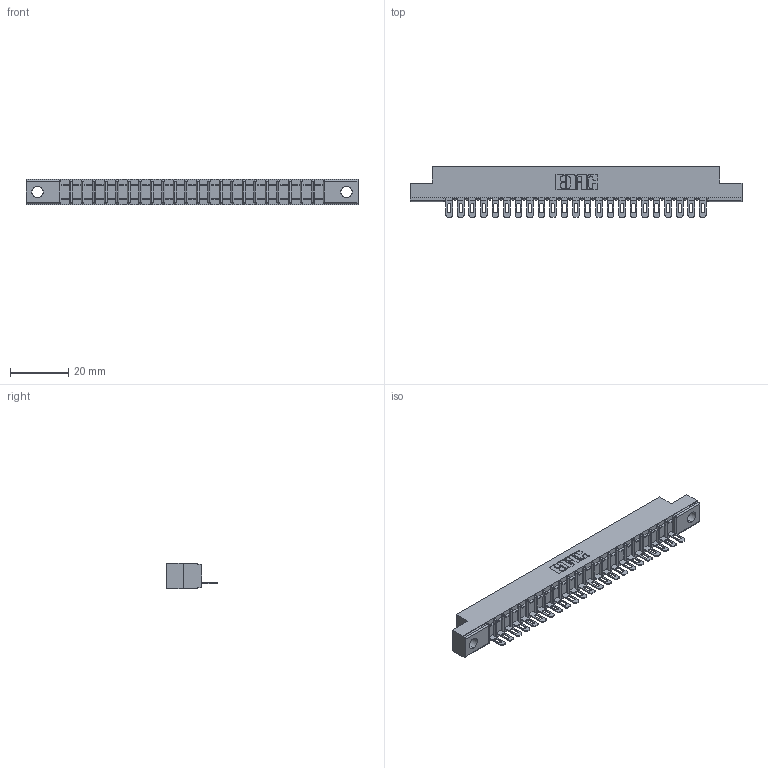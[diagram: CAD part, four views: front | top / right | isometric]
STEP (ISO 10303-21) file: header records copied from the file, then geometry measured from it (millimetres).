
FILE_DESCRIPTION (( 'STEP AP203' ), '1' );
FILE_NAME ('357-023-401-104.STEP', '2020-10-01T10:57:13', ( '' ), ( '' ), 'SwSTEP 2.0', 'SolidWorks 2020', '' );
FILE_SCHEMA (( 'CONFIG_CONTROL_DESIGN' ));
Length unit declared in the file: inch
Products named in the file (3): 307-290-002_501; 307 Part_.156 Dia Mounting Holes; 357-023-401-104
Assembly tree (24 placements, depth 2):
  357-023-401-104
    307 Part_.156 Dia Mounting Holes
    307-290-002_501  x23
Bounding box: 114.15 x 17.42 x 8.71 mm (x, y, z)
Volume: 7450.4 mm3; surface area: 13652.2 mm2
Topology: 24 solids, 24 shells, 1904 faces, 5833 edges, 3822 vertices
Faces by surface type: plane 1096, cylinder 760, sphere 48
Entity records: 23272 total; most frequent: CARTESIAN_POINT 3926, ORIENTED_EDGE 3914, DIRECTION 3819, EDGE_CURVE 1957, LINE 1493, VECTOR 1493, VERTEX_POINT 1270, AXIS2_PLACEMENT_3D 1163
